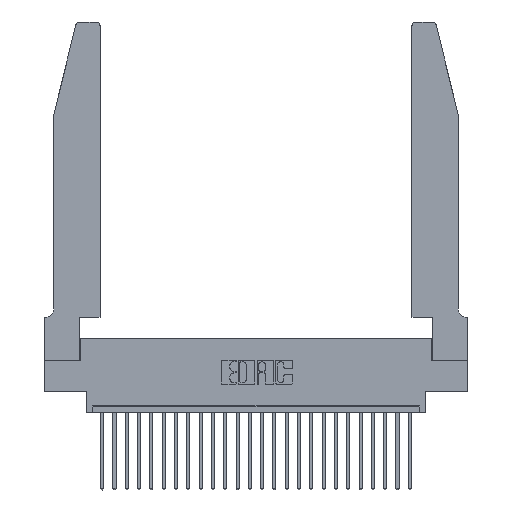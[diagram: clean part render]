
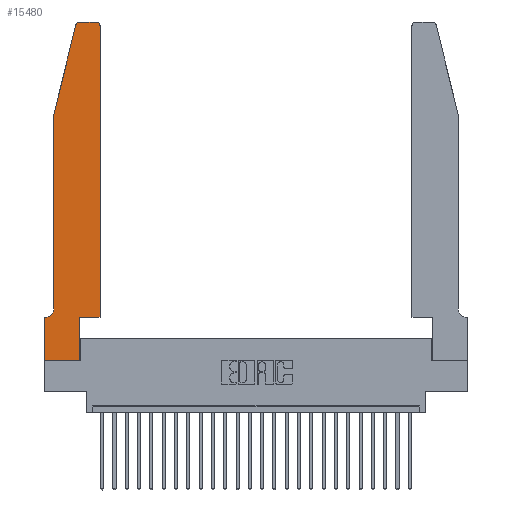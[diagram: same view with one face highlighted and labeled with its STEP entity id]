
A CAD part, top view. The second image highlights one B-rep face of the part: STEP entity #15480.
In plain terms, the highlighted planar face has unit normal (0, 0, 1).
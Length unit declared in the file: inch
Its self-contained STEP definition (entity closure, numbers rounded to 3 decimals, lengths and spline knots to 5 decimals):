
#286 = ORIENTED_EDGE ( 'NONE', *, *, #1578, .T. ) ;
#614 = LINE ( 'NONE', #905, #21861 ) ;
#674 = CARTESIAN_POINT ( 'NONE',  ( 0.0755, 2., 0.37 ) ) ;
#857 = VECTOR ( 'NONE', #23041, 39.37008 ) ;
#882 = LINE ( 'NONE', #3805, #20847 ) ;
#905 = CARTESIAN_POINT ( 'NONE',  ( 0.2865, 0.35, 0.37 ) ) ;
#1578 = EDGE_CURVE ( 'NONE', #10800, #24364, #4025, .T. ) ;
#1581 = ORIENTED_EDGE ( 'NONE', *, *, #13488, .T. ) ;
#2183 = LINE ( 'NONE', #674, #19220 ) ;
#2290 = VERTEX_POINT ( 'NONE', #17792 ) ;
#2436 = CARTESIAN_POINT ( 'NONE',  ( 0.0055, 0.35, 0.37 ) ) ;
#2594 = PLANE ( 'NONE',  #9544 ) ;
#2652 = CARTESIAN_POINT ( 'NONE',  ( 0., 0., 0.37 ) ) ;
#2742 = DIRECTION ( 'NONE',  ( 1., 0., 0. ) ) ;
#3236 = DIRECTION ( 'NONE',  ( 0., 0., -1. ) ) ;
#3342 = DIRECTION ( 'NONE',  ( 0., -1., 0. ) ) ;
#3805 = CARTESIAN_POINT ( 'NONE',  ( 0.0755, 0.35, 0.37 ) ) ;
#4025 = LINE ( 'NONE', #2652, #18481 ) ;
#4103 = DIRECTION ( 'NONE',  ( 1., 0., 0. ) ) ;
#4294 = CIRCLE ( 'NONE', #11688, 0.07 ) ;
#4590 = AXIS2_PLACEMENT_3D ( 'NONE', #7737, #7975, #4103 ) ;
#4811 = CARTESIAN_POINT ( 'NONE',  ( 0.284, 2.75, 0.37 ) ) ;
#5173 = CIRCLE ( 'NONE', #4590, 0.03 ) ;
#5246 = CARTESIAN_POINT ( 'NONE',  ( 0.4505, 0.35, 0.37 ) ) ;
#5778 = DIRECTION ( 'NONE',  ( -1., 0., 0. ) ) ;
#5902 = ORIENTED_EDGE ( 'NONE', *, *, #15674, .T. ) ;
#6182 = VERTEX_POINT ( 'NONE', #7850 ) ;
#6367 = EDGE_CURVE ( 'NONE', #25363, #25842, #5173, .T. ) ;
#6527 = CIRCLE ( 'NONE', #18941, 0.03 ) ;
#6683 = EDGE_CURVE ( 'NONE', #25215, #7204, #7085, .T. ) ;
#7085 = LINE ( 'NONE', #5246, #22559 ) ;
#7204 = VERTEX_POINT ( 'NONE', #8816 ) ;
#7737 = CARTESIAN_POINT ( 'NONE',  ( 0.284, 2.72, 0.37 ) ) ;
#7850 = CARTESIAN_POINT ( 'NONE',  ( 0.4205, 2.75, 0.37 ) ) ;
#7975 = DIRECTION ( 'NONE',  ( 0., 0., 1. ) ) ;
#8605 = VERTEX_POINT ( 'NONE', #16595 ) ;
#8816 = CARTESIAN_POINT ( 'NONE',  ( 0.4505, 2.72, 0.37 ) ) ;
#9171 = ORIENTED_EDGE ( 'NONE', *, *, #12089, .T. ) ;
#9247 = CARTESIAN_POINT ( 'NONE',  ( 0.4505, 0.35, 0.37 ) ) ;
#9301 = DIRECTION ( 'NONE',  ( 0., 1., 0. ) ) ;
#9544 = AXIS2_PLACEMENT_3D ( 'NONE', #20928, #14636, #12916 ) ;
#9586 = LINE ( 'NONE', #21057, #857 ) ;
#9903 = VECTOR ( 'NONE', #5778, 39.37008 ) ;
#10035 = LINE ( 'NONE', #11514, #19332 ) ;
#10221 = CARTESIAN_POINT ( 'NONE',  ( 0.4505, 0.35, 0.37 ) ) ;
#10800 = VERTEX_POINT ( 'NONE', #17854 ) ;
#10935 = DIRECTION ( 'NONE',  ( 0., -1., 0. ) ) ;
#11514 = CARTESIAN_POINT ( 'NONE',  ( 0., 0., 0.37 ) ) ;
#11688 = AXIS2_PLACEMENT_3D ( 'NONE', #19674, #3236, #23806 ) ;
#12089 = EDGE_CURVE ( 'NONE', #2290, #25215, #23553, .T. ) ;
#12295 = DIRECTION ( 'NONE',  ( 0., 0., 1. ) ) ;
#12793 = ORIENTED_EDGE ( 'NONE', *, *, #15131, .T. ) ;
#12916 = DIRECTION ( 'NONE',  ( 1., 0., 0. ) ) ;
#13435 = DIRECTION ( 'NONE',  ( 0., 1., 0. ) ) ;
#13488 = EDGE_CURVE ( 'NONE', #16810, #10800, #10035, .T. ) ;
#14039 = CARTESIAN_POINT ( 'NONE',  ( 0.25487, 2.72718, 0.37 ) ) ;
#14091 = LINE ( 'NONE', #24322, #9903 ) ;
#14636 = DIRECTION ( 'NONE',  ( 0., 0., 1. ) ) ;
#15087 = EDGE_CURVE ( 'NONE', #6182, #25363, #14091, .T. ) ;
#15131 = EDGE_CURVE ( 'NONE', #24237, #16810, #882, .T. ) ;
#15480 = ADVANCED_FACE ( 'NONE', ( #21802 ), #2594, .T. ) ;
#15488 = EDGE_CURVE ( 'NONE', #23308, #8605, #2183, .T. ) ;
#15510 = DIRECTION ( 'NONE',  ( 1., 0., 0. ) ) ;
#15674 = EDGE_CURVE ( 'NONE', #25842, #23308, #9586, .T. ) ;
#16595 = CARTESIAN_POINT ( 'NONE',  ( 0.0755, 0.42, 0.37 ) ) ;
#16810 = VERTEX_POINT ( 'NONE', #20454 ) ;
#16814 = VECTOR ( 'NONE', #15510, 39.37008 ) ;
#16896 = ORIENTED_EDGE ( 'NONE', *, *, #15087, .T. ) ;
#17500 = CARTESIAN_POINT ( 'NONE',  ( 0.0755, 2., 0.37 ) ) ;
#17792 = CARTESIAN_POINT ( 'NONE',  ( 0.2865, 0.35, 0.37 ) ) ;
#17854 = CARTESIAN_POINT ( 'NONE',  ( 0., 0., 0.37 ) ) ;
#18407 = CARTESIAN_POINT ( 'NONE',  ( 0.4205, 2.72, 0.37 ) ) ;
#18481 = VECTOR ( 'NONE', #2742, 39.37008 ) ;
#18584 = DIRECTION ( 'NONE',  ( 1., 0., 0. ) ) ;
#18941 = AXIS2_PLACEMENT_3D ( 'NONE', #18407, #12295, #18584 ) ;
#19044 = CARTESIAN_POINT ( 'NONE',  ( 0.2865, 0., 0.37 ) ) ;
#19220 = VECTOR ( 'NONE', #10935, 39.37008 ) ;
#19332 = VECTOR ( 'NONE', #3342, 39.37008 ) ;
#19674 = CARTESIAN_POINT ( 'NONE',  ( 0.0055, 0.42, 0.37 ) ) ;
#20251 = DIRECTION ( 'NONE',  ( -1., 0., 0. ) ) ;
#20454 = CARTESIAN_POINT ( 'NONE',  ( 0., 0.35, 0.37 ) ) ;
#20847 = VECTOR ( 'NONE', #20251, 39.37008 ) ;
#20928 = CARTESIAN_POINT ( 'NONE',  ( 0., 0.35, 0.37 ) ) ;
#20963 = ORIENTED_EDGE ( 'NONE', *, *, #25564, .T. ) ;
#21057 = CARTESIAN_POINT ( 'NONE',  ( 0.0755, 2., 0.37 ) ) ;
#21802 = FACE_OUTER_BOUND ( 'NONE', #26066, .T. ) ;
#21861 = VECTOR ( 'NONE', #9301, 39.37008 ) ;
#22386 = ORIENTED_EDGE ( 'NONE', *, *, #15488, .T. ) ;
#22536 = ORIENTED_EDGE ( 'NONE', *, *, #22725, .T. ) ;
#22559 = VECTOR ( 'NONE', #13435, 39.37008 ) ;
#22725 = EDGE_CURVE ( 'NONE', #8605, #24237, #4294, .T. ) ;
#22973 = EDGE_CURVE ( 'NONE', #7204, #6182, #6527, .T. ) ;
#23041 = DIRECTION ( 'NONE',  ( -0.239, -0.971, 0. ) ) ;
#23308 = VERTEX_POINT ( 'NONE', #17500 ) ;
#23553 = LINE ( 'NONE', #9247, #16814 ) ;
#23806 = DIRECTION ( 'NONE',  ( -1., 0., 0. ) ) ;
#24237 = VERTEX_POINT ( 'NONE', #2436 ) ;
#24322 = CARTESIAN_POINT ( 'NONE',  ( 0.2605, 2.75, 0.37 ) ) ;
#24364 = VERTEX_POINT ( 'NONE', #19044 ) ;
#24433 = ORIENTED_EDGE ( 'NONE', *, *, #6367, .T. ) ;
#25215 = VERTEX_POINT ( 'NONE', #10221 ) ;
#25294 = ORIENTED_EDGE ( 'NONE', *, *, #6683, .T. ) ;
#25363 = VERTEX_POINT ( 'NONE', #4811 ) ;
#25564 = EDGE_CURVE ( 'NONE', #24364, #2290, #614, .T. ) ;
#25842 = VERTEX_POINT ( 'NONE', #14039 ) ;
#26066 = EDGE_LOOP ( 'NONE', ( #16896, #24433, #5902, #22386, #22536, #12793, #1581, #286, #20963, #9171, #25294, #26402 ) ) ;
#26402 = ORIENTED_EDGE ( 'NONE', *, *, #22973, .T. ) ;
